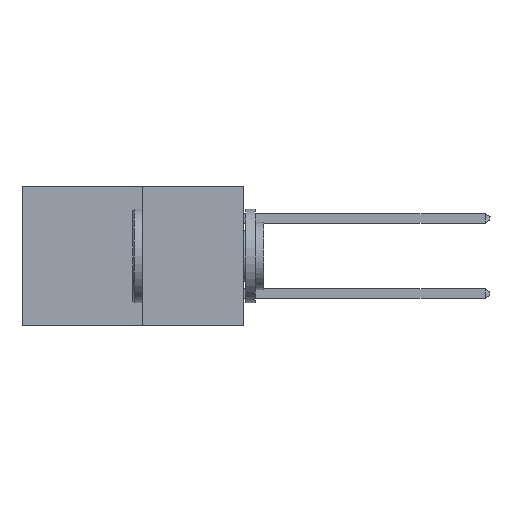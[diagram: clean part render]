
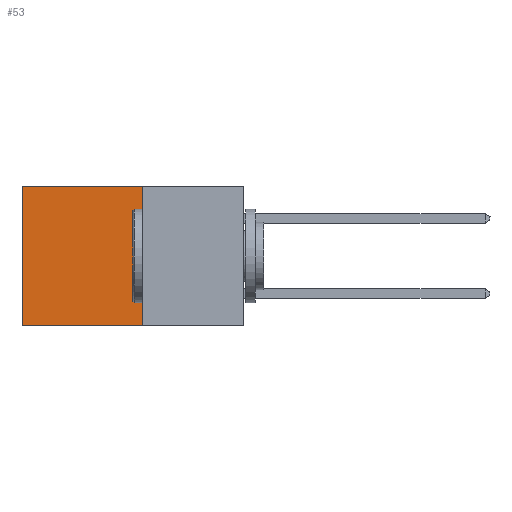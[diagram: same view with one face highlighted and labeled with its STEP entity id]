
A CAD part, left-side view. The second image highlights one B-rep face of the part: STEP entity #53.
In plain terms, the highlighted planar face has unit normal (-1, 0, 0).
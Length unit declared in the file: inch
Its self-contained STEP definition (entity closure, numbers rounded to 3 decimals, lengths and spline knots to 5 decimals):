
#53 = ADVANCED_FACE ( 'NONE', ( #5088 ), #3969, .F. ) ;
#131 = EDGE_CURVE ( 'NONE', #9817, #4311, #8436, .T. ) ;
#500 = DIRECTION ( 'NONE',  ( 0., 0., -1. ) ) ;
#650 = DIRECTION ( 'NONE',  ( 0., 1., 0. ) ) ;
#672 = EDGE_CURVE ( 'NONE', #9817, #7739, #6987, .T. ) ;
#1013 = DIRECTION ( 'NONE',  ( 0., 1., 0. ) ) ;
#1552 = ORIENTED_EDGE ( 'NONE', *, *, #9158, .F. ) ;
#1962 = LINE ( 'NONE', #9482, #4129 ) ;
#2493 = ORIENTED_EDGE ( 'NONE', *, *, #131, .T. ) ;
#2740 = DIRECTION ( 'NONE',  ( 0., 0., -1. ) ) ;
#2806 = DIRECTION ( 'NONE',  ( 1., 0., 0. ) ) ;
#3455 = VERTEX_POINT ( 'NONE', #5294 ) ;
#3580 = CARTESIAN_POINT ( 'NONE',  ( 0.277, 0.27, -0.37 ) ) ;
#3969 = PLANE ( 'NONE',  #8893 ) ;
#4012 = VECTOR ( 'NONE', #1013, 39.37008 ) ;
#4058 = CARTESIAN_POINT ( 'NONE',  ( 0.277, 0.59, 0. ) ) ;
#4129 = VECTOR ( 'NONE', #2740, 39.37008 ) ;
#4195 = CARTESIAN_POINT ( 'NONE',  ( 0.277, 0.27, 0. ) ) ;
#4311 = VERTEX_POINT ( 'NONE', #4058 ) ;
#5088 = FACE_OUTER_BOUND ( 'NONE', #8645, .T. ) ;
#5294 = CARTESIAN_POINT ( 'NONE',  ( 0.277, 0.59, -0.37 ) ) ;
#5520 = EDGE_CURVE ( 'NONE', #4311, #3455, #1962, .T. ) ;
#5633 = ORIENTED_EDGE ( 'NONE', *, *, #5520, .T. ) ;
#5650 = LINE ( 'NONE', #7706, #7325 ) ;
#5690 = CARTESIAN_POINT ( 'NONE',  ( 0.277, 0.27, -0.37 ) ) ;
#5955 = ORIENTED_EDGE ( 'NONE', *, *, #672, .F. ) ;
#6987 = LINE ( 'NONE', #9082, #8675 ) ;
#7325 = VECTOR ( 'NONE', #650, 39.37008 ) ;
#7706 = CARTESIAN_POINT ( 'NONE',  ( 0.277, 0.27, -0.37 ) ) ;
#7739 = VERTEX_POINT ( 'NONE', #3580 ) ;
#8138 = DIRECTION ( 'NONE',  ( 0., 0., -1. ) ) ;
#8436 = LINE ( 'NONE', #10196, #4012 ) ;
#8645 = EDGE_LOOP ( 'NONE', ( #5633, #1552, #5955, #2493 ) ) ;
#8675 = VECTOR ( 'NONE', #500, 39.37008 ) ;
#8893 = AXIS2_PLACEMENT_3D ( 'NONE', #5690, #2806, #8138 ) ;
#9082 = CARTESIAN_POINT ( 'NONE',  ( 0.277, 0.27, -0.37 ) ) ;
#9158 = EDGE_CURVE ( 'NONE', #7739, #3455, #5650, .T. ) ;
#9482 = CARTESIAN_POINT ( 'NONE',  ( 0.277, 0.59, -0.37 ) ) ;
#9817 = VERTEX_POINT ( 'NONE', #4195 ) ;
#10196 = CARTESIAN_POINT ( 'NONE',  ( 0.277, 0.27, 0. ) ) ;
